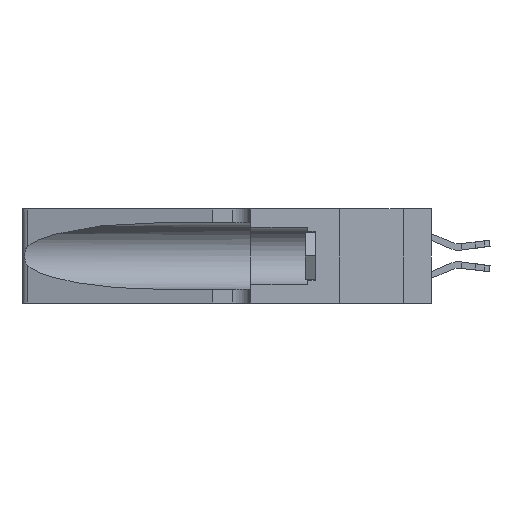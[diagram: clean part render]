
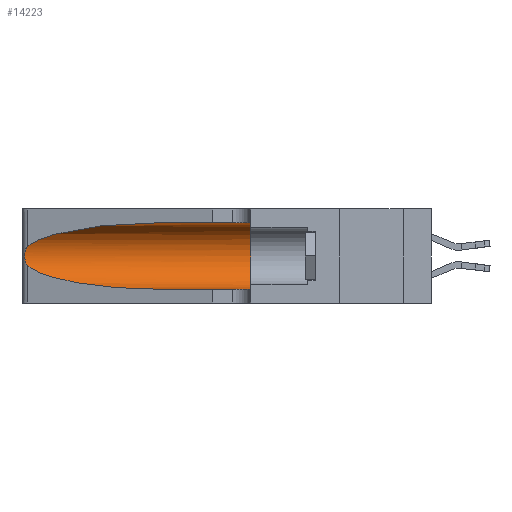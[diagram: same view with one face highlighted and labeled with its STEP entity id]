
A CAD part, left-side view. The second image highlights one B-rep face of the part: STEP entity #14223.
In plain terms, the highlighted cylindrical face has radius 3.308 mm (diameter 6.617 mm), a partial arc.
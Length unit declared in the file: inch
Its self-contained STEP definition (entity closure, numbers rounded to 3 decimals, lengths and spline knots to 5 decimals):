
#79 = CARTESIAN_POINT ( 'NONE',  ( 0.26075, 1.23896, 0.178 ) ) ;
#321 = DIRECTION ( 'NONE',  ( 0., 0., -1. ) ) ;
#322 = ORIENTED_EDGE ( 'NONE', *, *, #6982, .T. ) ;
#360 = CARTESIAN_POINT ( 'NONE',  ( 0.25487, 1.22718, 0.22369 ) ) ;
#1147 = EDGE_CURVE ( 'NONE', #14252, #12912, #15275, .T. ) ;
#2604 = CARTESIAN_POINT ( 'NONE',  ( 0.25487, 1.22718, 0.22369 ) ) ;
#2738 = CARTESIAN_POINT ( 'NONE',  ( 0.2373, 1.15595, 0.28018 ) ) ;
#3363 = CARTESIAN_POINT ( 'NONE',  ( 0.25487, 1.22718, 0.22369 ) ) ;
#3379 = CARTESIAN_POINT ( 'NONE',  ( 0.1305, 0.35, 0.185 ) ) ;
#4236 = AXIS2_PLACEMENT_3D ( 'NONE', #3379, #6585, #14552 ) ;
#4285 = CARTESIAN_POINT ( 'NONE',  ( 0.1305, 0.72297, 0.31525 ) ) ;
#4811 = CARTESIAN_POINT ( 'NONE',  ( 0.25856, 1.23593, 0.16098 ) ) ;
#5108 = CARTESIAN_POINT ( 'NONE',  ( 0.1305, 1.61858, 0.185 ) ) ;
#5377 =( BOUNDED_CURVE ( )  B_SPLINE_CURVE ( 3, ( #17704, #16161, #8370, #19510 ),
 .UNSPECIFIED., .F., .F. ) 
 B_SPLINE_CURVE_WITH_KNOTS ( ( 4, 4 ),
 ( 3.44316, 4.71239 ),
 .UNSPECIFIED. ) 
 CURVE ( )  GEOMETRIC_REPRESENTATION_ITEM ( )  RATIONAL_B_SPLINE_CURVE ( ( 1., 0.87, 0.87, 1. ) ) 
 REPRESENTATION_ITEM ( '' )  );
#5395 = EDGE_CURVE ( 'NONE', #8585, #5911, #5377, .T. ) ;
#5911 = VERTEX_POINT ( 'NONE', #16833 ) ;
#6567 = CARTESIAN_POINT ( 'NONE',  ( 0.25789, 1.23486, 0.15765 ) ) ;
#6585 = DIRECTION ( 'NONE',  ( 0., 1., 0. ) ) ;
#6856 = DIRECTION ( 'NONE',  ( 0., -1., 0. ) ) ;
#6982 = EDGE_CURVE ( 'NONE', #14252, #9386, #8838, .T. ) ;
#7440 = EDGE_LOOP ( 'NONE', ( #322, #11450, #8028, #12837, #15351, #8430 ) ) ;
#7447 = DIRECTION ( 'NONE',  ( 0., -1., 0. ) ) ;
#7967 = CARTESIAN_POINT ( 'NONE',  ( 0.25555, 1.22994, 0.2215 ) ) ;
#8028 = ORIENTED_EDGE ( 'NONE', *, *, #5395, .T. ) ;
#8123 = CARTESIAN_POINT ( 'NONE',  ( 0.26075, 1.23896, 0.19203 ) ) ;
#8135 = DIRECTION ( 'NONE',  ( 0., -1., 0. ) ) ;
#8248 = CARTESIAN_POINT ( 'NONE',  ( 0.25487, 1.22718, 0.14631 ) ) ;
#8273 = LINE ( 'NONE', #10824, #19745 ) ;
#8370 = CARTESIAN_POINT ( 'NONE',  ( 0.18966, 0.96281, 0.05475 ) ) ;
#8430 = ORIENTED_EDGE ( 'NONE', *, *, #1147, .F. ) ;
#8585 = VERTEX_POINT ( 'NONE', #10784 ) ;
#8838 =( BOUNDED_CURVE ( )  B_SPLINE_CURVE ( 3, ( #4285, #16953, #2738, #2604 ),
 .UNSPECIFIED., .F., .T. ) 
 B_SPLINE_CURVE_WITH_KNOTS ( ( 4, 4 ),
 ( 1.5708, 2.84003 ),
 .UNSPECIFIED. ) 
 CURVE ( )  GEOMETRIC_REPRESENTATION_ITEM ( )  RATIONAL_B_SPLINE_CURVE ( ( 1., 0.87, 0.87, 1. ) ) 
 REPRESENTATION_ITEM ( '' )  );
#9386 = VERTEX_POINT ( 'NONE', #360 ) ;
#9748 = EDGE_CURVE ( 'NONE', #5911, #9943, #8273, .T. ) ;
#9792 = CARTESIAN_POINT ( 'NONE',  ( 0.25854, 1.2359, 0.20912 ) ) ;
#9857 = CYLINDRICAL_SURFACE ( 'NONE', #16124, 0.13025 ) ;
#9943 = VERTEX_POINT ( 'NONE', #14748 ) ;
#10567 = VECTOR ( 'NONE', #8135, 39.37008 ) ;
#10784 = CARTESIAN_POINT ( 'NONE',  ( 0.25487, 1.22718, 0.14631 ) ) ;
#10824 = CARTESIAN_POINT ( 'NONE',  ( 0.1305, 1.61858, 0.05475 ) ) ;
#10862 = FACE_OUTER_BOUND ( 'NONE', #7440, .T. ) ;
#11212 = CARTESIAN_POINT ( 'NONE',  ( 0.25639, 1.23184, 0.21858 ) ) ;
#11450 = ORIENTED_EDGE ( 'NONE', *, *, #19446, .T. ) ;
#11685 = B_SPLINE_CURVE_WITH_KNOTS ( 'NONE', 3,
 ( #3363, #7967, #11212, #19112, #9792, #16055, #8123, #79, #14533, #4811, #6567, #12805, #17727, #8248 ),
 .UNSPECIFIED., .F., .F.,
 ( 4, 2, 2, 2, 2, 2, 4 ),
 ( 0., 0.00027, 0.00053, 0.00107, 0.0016, 0.00187, 0.00214 ),
 .UNSPECIFIED. ) ;
#12805 = CARTESIAN_POINT ( 'NONE',  ( 0.25639, 1.23186, 0.15144 ) ) ;
#12837 = ORIENTED_EDGE ( 'NONE', *, *, #9748, .T. ) ;
#12912 = VERTEX_POINT ( 'NONE', #17895 ) ;
#14155 = EDGE_CURVE ( 'NONE', #12912, #9943, #17080, .T. ) ;
#14223 = ADVANCED_FACE ( 'NONE', ( #10862 ), #9857, .F. ) ;
#14252 = VERTEX_POINT ( 'NONE', #17933 ) ;
#14533 = CARTESIAN_POINT ( 'NONE',  ( 0.26017, 1.23833, 0.17102 ) ) ;
#14552 = DIRECTION ( 'NONE',  ( 0., 0., 1. ) ) ;
#14748 = CARTESIAN_POINT ( 'NONE',  ( 0.1305, 0.35, 0.05475 ) ) ;
#15275 = LINE ( 'NONE', #15782, #10567 ) ;
#15351 = ORIENTED_EDGE ( 'NONE', *, *, #14155, .F. ) ;
#15782 = CARTESIAN_POINT ( 'NONE',  ( 0.1305, 1.61858, 0.31525 ) ) ;
#16055 = CARTESIAN_POINT ( 'NONE',  ( 0.26018, 1.23835, 0.19895 ) ) ;
#16124 = AXIS2_PLACEMENT_3D ( 'NONE', #5108, #6856, #321 ) ;
#16161 = CARTESIAN_POINT ( 'NONE',  ( 0.2373, 1.15595, 0.08982 ) ) ;
#16833 = CARTESIAN_POINT ( 'NONE',  ( 0.1305, 0.72297, 0.05475 ) ) ;
#16953 = CARTESIAN_POINT ( 'NONE',  ( 0.18966, 0.96281, 0.31525 ) ) ;
#17080 = CIRCLE ( 'NONE', #4236, 0.13025 ) ;
#17704 = CARTESIAN_POINT ( 'NONE',  ( 0.25487, 1.22718, 0.14631 ) ) ;
#17727 = CARTESIAN_POINT ( 'NONE',  ( 0.25555, 1.22993, 0.14849 ) ) ;
#17895 = CARTESIAN_POINT ( 'NONE',  ( 0.1305, 0.35, 0.31525 ) ) ;
#17933 = CARTESIAN_POINT ( 'NONE',  ( 0.1305, 0.72297, 0.31525 ) ) ;
#19112 = CARTESIAN_POINT ( 'NONE',  ( 0.25787, 1.23484, 0.2124 ) ) ;
#19446 = EDGE_CURVE ( 'NONE', #9386, #8585, #11685, .T. ) ;
#19510 = CARTESIAN_POINT ( 'NONE',  ( 0.1305, 0.72297, 0.05475 ) ) ;
#19745 = VECTOR ( 'NONE', #7447, 39.37008 ) ;
